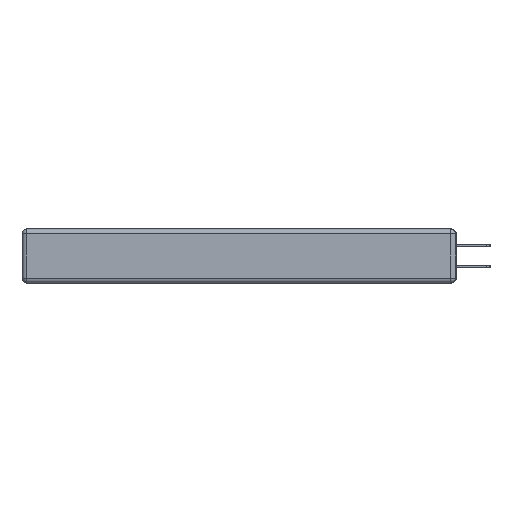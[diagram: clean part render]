
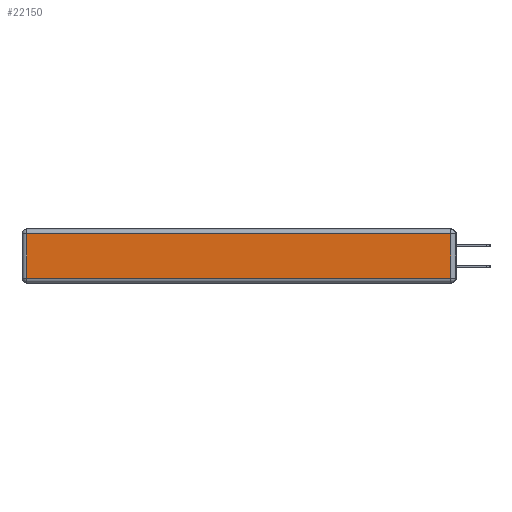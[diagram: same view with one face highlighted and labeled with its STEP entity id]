
A CAD part, left-side view. The second image highlights one B-rep face of the part: STEP entity #22150.
In plain terms, the highlighted planar face has unit normal (-1, 0, 0).
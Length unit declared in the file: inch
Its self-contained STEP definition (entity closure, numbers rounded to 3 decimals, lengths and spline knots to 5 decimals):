
#575 = CARTESIAN_POINT ( 'NONE',  ( 0., 2.72, -0.03 ) ) ;
#657 = VERTEX_POINT ( 'NONE', #575 ) ;
#1417 = AXIS2_PLACEMENT_3D ( 'NONE', #3458, #20390, #16296 ) ;
#1781 = LINE ( 'NONE', #20865, #21606 ) ;
#1900 = LINE ( 'NONE', #10510, #19645 ) ;
#2080 = ORIENTED_EDGE ( 'NONE', *, *, #15720, .T. ) ;
#3458 = CARTESIAN_POINT ( 'NONE',  ( 0., 0., -0.343 ) ) ;
#4883 = VECTOR ( 'NONE', #22419, 39.37008 ) ;
#4974 = DIRECTION ( 'NONE',  ( 0., -1., 0. ) ) ;
#5678 = CARTESIAN_POINT ( 'NONE',  ( 0., 2.75, -0.03 ) ) ;
#5930 = ORIENTED_EDGE ( 'NONE', *, *, #18094, .T. ) ;
#6608 = DIRECTION ( 'NONE',  ( 0., 0., 1. ) ) ;
#6889 = CARTESIAN_POINT ( 'NONE',  ( 0., 0.03, -0.03 ) ) ;
#6974 = CARTESIAN_POINT ( 'NONE',  ( 0., 2.72, -0.313 ) ) ;
#9859 = CARTESIAN_POINT ( 'NONE',  ( 0., 2.72, -0.343 ) ) ;
#10510 = CARTESIAN_POINT ( 'NONE',  ( 0., 0., -0.313 ) ) ;
#11683 = ORIENTED_EDGE ( 'NONE', *, *, #20501, .T. ) ;
#14508 = FACE_OUTER_BOUND ( 'NONE', #20846, .T. ) ;
#14575 = PLANE ( 'NONE',  #1417 ) ;
#14829 = VERTEX_POINT ( 'NONE', #16495 ) ;
#15720 = EDGE_CURVE ( 'NONE', #657, #18727, #22053, .T. ) ;
#16296 = DIRECTION ( 'NONE',  ( 0., 0., 1. ) ) ;
#16495 = CARTESIAN_POINT ( 'NONE',  ( 0., 0.03, -0.313 ) ) ;
#16863 = LINE ( 'NONE', #5678, #4883 ) ;
#17134 = ORIENTED_EDGE ( 'NONE', *, *, #22260, .T. ) ;
#17557 = DIRECTION ( 'NONE',  ( 0., 0., -1. ) ) ;
#18094 = EDGE_CURVE ( 'NONE', #18727, #14829, #1900, .T. ) ;
#18727 = VERTEX_POINT ( 'NONE', #6974 ) ;
#18830 = VECTOR ( 'NONE', #17557, 39.37008 ) ;
#19645 = VECTOR ( 'NONE', #4974, 39.37008 ) ;
#20390 = DIRECTION ( 'NONE',  ( -1., 0., 0. ) ) ;
#20501 = EDGE_CURVE ( 'NONE', #14829, #21704, #1781, .T. ) ;
#20846 = EDGE_LOOP ( 'NONE', ( #5930, #11683, #17134, #2080 ) ) ;
#20865 = CARTESIAN_POINT ( 'NONE',  ( 0., 0.03, -0.343 ) ) ;
#21606 = VECTOR ( 'NONE', #6608, 39.37008 ) ;
#21704 = VERTEX_POINT ( 'NONE', #6889 ) ;
#22053 = LINE ( 'NONE', #9859, #18830 ) ;
#22150 = ADVANCED_FACE ( 'NONE', ( #14508 ), #14575, .T. ) ;
#22260 = EDGE_CURVE ( 'NONE', #21704, #657, #16863, .T. ) ;
#22419 = DIRECTION ( 'NONE',  ( 0., 1., 0. ) ) ;
